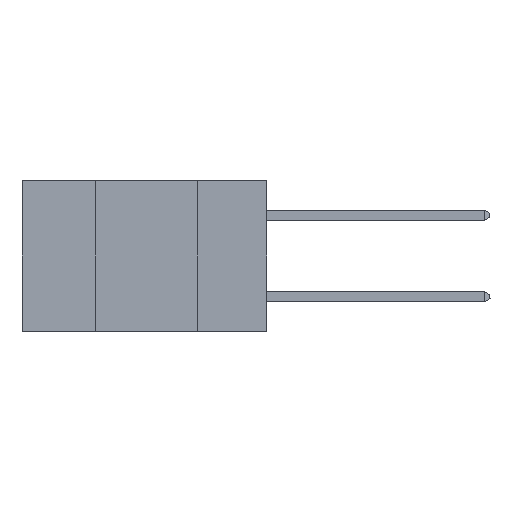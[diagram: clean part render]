
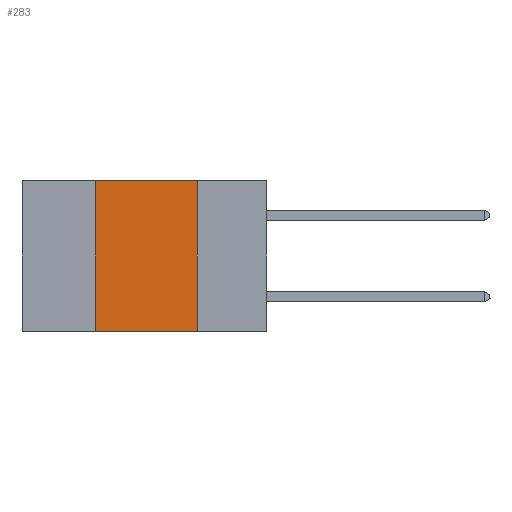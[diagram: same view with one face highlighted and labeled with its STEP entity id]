
A CAD part, left-side view. The second image highlights one B-rep face of the part: STEP entity #283.
In plain terms, the highlighted planar face has unit normal (-1, 0, 0).
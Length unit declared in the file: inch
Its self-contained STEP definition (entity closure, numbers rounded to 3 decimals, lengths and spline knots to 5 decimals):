
#283 = ADVANCED_FACE ( 'NONE', ( #26344 ), #1025, .F. ) ;
#1025 = PLANE ( 'NONE',  #35530 ) ;
#1848 = CARTESIAN_POINT ( 'NONE',  ( 0., 0.6, -0.37 ) ) ;
#2195 = LINE ( 'NONE', #1848, #11283 ) ;
#2838 = VERTEX_POINT ( 'NONE', #12182 ) ;
#3251 = VERTEX_POINT ( 'NONE', #20692 ) ;
#5004 = CARTESIAN_POINT ( 'NONE',  ( 0., 0.42, 0. ) ) ;
#5228 = DIRECTION ( 'NONE',  ( 0., -1., 0. ) ) ;
#5352 = CARTESIAN_POINT ( 'NONE',  ( 0., 0.6, 0. ) ) ;
#5928 = ORIENTED_EDGE ( 'NONE', *, *, #26194, .F. ) ;
#7084 = ORIENTED_EDGE ( 'NONE', *, *, #31514, .T. ) ;
#9439 = EDGE_CURVE ( 'NONE', #31120, #2838, #33824, .T. ) ;
#10448 = EDGE_LOOP ( 'NONE', ( #5928, #19532, #35008, #7084 ) ) ;
#11283 = VECTOR ( 'NONE', #16387, 39.37008 ) ;
#12182 = CARTESIAN_POINT ( 'NONE',  ( 0., 0.17, 0. ) ) ;
#12520 = DIRECTION ( 'NONE',  ( 1., 0., 0. ) ) ;
#14253 = CARTESIAN_POINT ( 'NONE',  ( 0., 0.42, -0.37 ) ) ;
#15558 = DIRECTION ( 'NONE',  ( 0., 0., -1. ) ) ;
#16387 = DIRECTION ( 'NONE',  ( 0., -1., 0. ) ) ;
#18449 = DIRECTION ( 'NONE',  ( 0., 0., 1. ) ) ;
#19013 = EDGE_CURVE ( 'NONE', #28970, #31120, #36785, .T. ) ;
#19532 = ORIENTED_EDGE ( 'NONE', *, *, #9439, .F. ) ;
#20692 = CARTESIAN_POINT ( 'NONE',  ( 0., 0.17, -0.37 ) ) ;
#20976 = CARTESIAN_POINT ( 'NONE',  ( 0., 0.42, 0. ) ) ;
#21404 = CARTESIAN_POINT ( 'NONE',  ( 0., 0.6, 0. ) ) ;
#24123 = VECTOR ( 'NONE', #36697, 39.37008 ) ;
#26107 = VECTOR ( 'NONE', #5228, 39.37008 ) ;
#26194 = EDGE_CURVE ( 'NONE', #2838, #3251, #29568, .T. ) ;
#26344 = FACE_OUTER_BOUND ( 'NONE', #10448, .T. ) ;
#28970 = VERTEX_POINT ( 'NONE', #14253 ) ;
#29568 = LINE ( 'NONE', #33896, #24123 ) ;
#31120 = VERTEX_POINT ( 'NONE', #5004 ) ;
#31514 = EDGE_CURVE ( 'NONE', #28970, #3251, #2195, .T. ) ;
#33824 = LINE ( 'NONE', #5352, #26107 ) ;
#33896 = CARTESIAN_POINT ( 'NONE',  ( 0., 0.17, 0. ) ) ;
#35008 = ORIENTED_EDGE ( 'NONE', *, *, #19013, .F. ) ;
#35530 = AXIS2_PLACEMENT_3D ( 'NONE', #21404, #12520, #15558 ) ;
#35848 = VECTOR ( 'NONE', #18449, 39.37008 ) ;
#36697 = DIRECTION ( 'NONE',  ( 0., 0., -1. ) ) ;
#36785 = LINE ( 'NONE', #20976, #35848 ) ;
